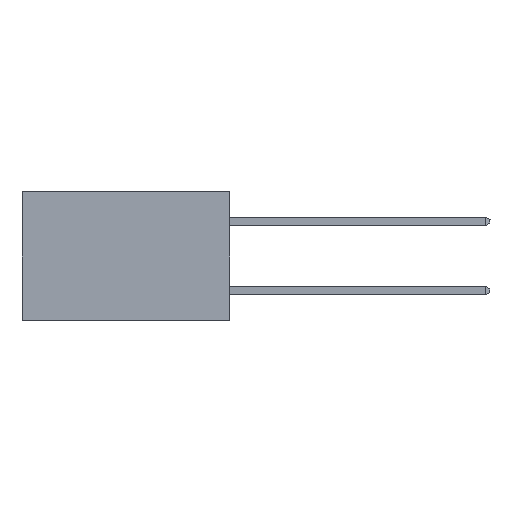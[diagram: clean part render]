
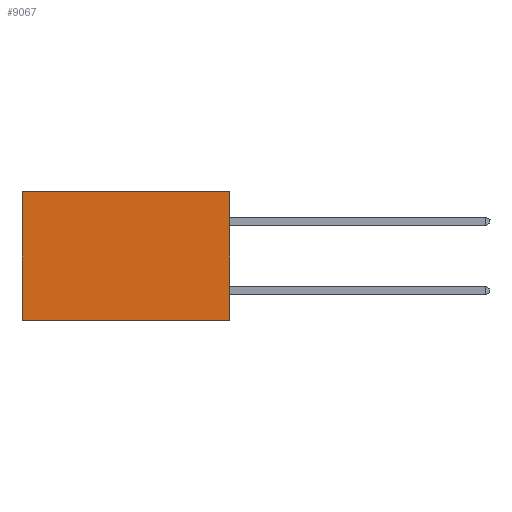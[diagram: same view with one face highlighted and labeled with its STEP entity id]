
A CAD part, left-side view. The second image highlights one B-rep face of the part: STEP entity #9067.
In plain terms, the highlighted planar face has unit normal (-1, 0, 0).
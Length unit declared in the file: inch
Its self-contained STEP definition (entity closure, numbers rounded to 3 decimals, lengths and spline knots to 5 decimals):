
#318 = CARTESIAN_POINT ( 'NONE',  ( 0.2615, 0., -0.37 ) ) ;
#957 = CARTESIAN_POINT ( 'NONE',  ( 0.2615, 0.6, -0.37 ) ) ;
#1019 = CARTESIAN_POINT ( 'NONE',  ( 0.2615, 0., 0. ) ) ;
#1058 = DIRECTION ( 'NONE',  ( 0., 0., -1. ) ) ;
#1063 = DIRECTION ( 'NONE',  ( 0., 0., -1. ) ) ;
#1089 = VECTOR ( 'NONE', #1063, 39.37008 ) ;
#1345 = ORIENTED_EDGE ( 'NONE', *, *, #18639, .T. ) ;
#2276 = EDGE_CURVE ( 'NONE', #18278, #12533, #13793, .T. ) ;
#3074 = VECTOR ( 'NONE', #7200, 39.37008 ) ;
#3440 = ORIENTED_EDGE ( 'NONE', *, *, #4701, .T. ) ;
#3692 = VECTOR ( 'NONE', #14950, 39.37008 ) ;
#4701 = EDGE_CURVE ( 'NONE', #18278, #5867, #19341, .T. ) ;
#4943 = ORIENTED_EDGE ( 'NONE', *, *, #2276, .F. ) ;
#5867 = VERTEX_POINT ( 'NONE', #6221 ) ;
#5871 = CARTESIAN_POINT ( 'NONE',  ( 0.2615, 0., -0.37 ) ) ;
#6221 = CARTESIAN_POINT ( 'NONE',  ( 0.2615, 0.6, 0. ) ) ;
#7200 = DIRECTION ( 'NONE',  ( 0., 1., 0. ) ) ;
#7302 = VECTOR ( 'NONE', #1058, 39.37008 ) ;
#8029 = FACE_OUTER_BOUND ( 'NONE', #10793, .T. ) ;
#8227 = PLANE ( 'NONE',  #10570 ) ;
#8537 = ORIENTED_EDGE ( 'NONE', *, *, #16292, .F. ) ;
#9067 = ADVANCED_FACE ( 'NONE', ( #8029 ), #8227, .F. ) ;
#9219 = VERTEX_POINT ( 'NONE', #16598 ) ;
#10570 = AXIS2_PLACEMENT_3D ( 'NONE', #318, #14472, #12741 ) ;
#10793 = EDGE_LOOP ( 'NONE', ( #1345, #8537, #4943, #3440 ) ) ;
#12137 = LINE ( 'NONE', #957, #7302 ) ;
#12533 = VERTEX_POINT ( 'NONE', #19514 ) ;
#12741 = DIRECTION ( 'NONE',  ( 0., 0., -1. ) ) ;
#13612 = CARTESIAN_POINT ( 'NONE',  ( 0.2615, 0., 0. ) ) ;
#13793 = LINE ( 'NONE', #19792, #1089 ) ;
#14472 = DIRECTION ( 'NONE',  ( 1., 0., 0. ) ) ;
#14950 = DIRECTION ( 'NONE',  ( 0., 1., 0. ) ) ;
#15044 = LINE ( 'NONE', #5871, #3692 ) ;
#16292 = EDGE_CURVE ( 'NONE', #12533, #9219, #15044, .T. ) ;
#16598 = CARTESIAN_POINT ( 'NONE',  ( 0.2615, 0.6, -0.37 ) ) ;
#18278 = VERTEX_POINT ( 'NONE', #13612 ) ;
#18639 = EDGE_CURVE ( 'NONE', #5867, #9219, #12137, .T. ) ;
#19341 = LINE ( 'NONE', #1019, #3074 ) ;
#19514 = CARTESIAN_POINT ( 'NONE',  ( 0.2615, 0., -0.37 ) ) ;
#19792 = CARTESIAN_POINT ( 'NONE',  ( 0.2615, 0., -0.37 ) ) ;
